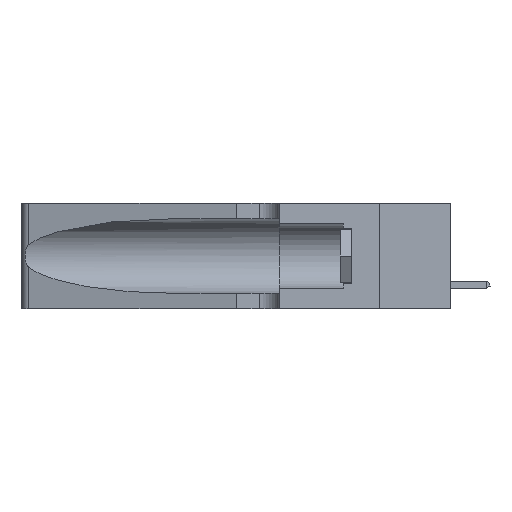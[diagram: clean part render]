
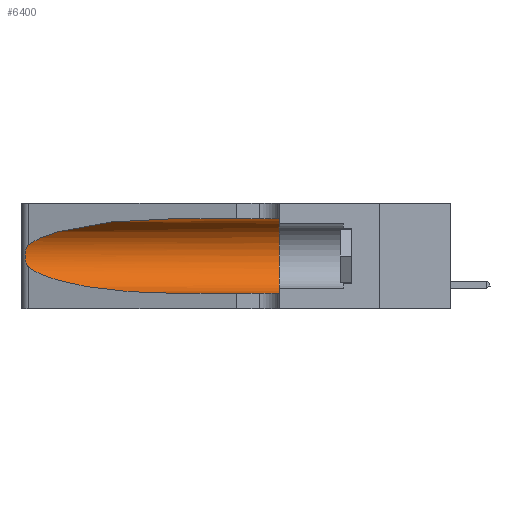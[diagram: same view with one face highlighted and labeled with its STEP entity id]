
A CAD part, left-side view. The second image highlights one B-rep face of the part: STEP entity #6400.
In plain terms, the highlighted cylindrical face has radius 3.308 mm (diameter 6.617 mm), a partial arc.
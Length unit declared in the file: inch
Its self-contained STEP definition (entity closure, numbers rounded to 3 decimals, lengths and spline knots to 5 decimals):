
#221 = CARTESIAN_POINT ( 'NONE',  ( 0.25555, 1.22993, 0.14849 ) ) ;
#281 = CARTESIAN_POINT ( 'NONE',  ( 0.25487, 1.22718, 0.22369 ) ) ;
#1464 = CARTESIAN_POINT ( 'NONE',  ( 0.25789, 1.23486, 0.15765 ) ) ;
#1633 = ORIENTED_EDGE ( 'NONE', *, *, #9034, .F. ) ;
#2254 = ORIENTED_EDGE ( 'NONE', *, *, #24382, .T. ) ;
#2431 = FACE_OUTER_BOUND ( 'NONE', #9905, .T. ) ;
#2759 = CARTESIAN_POINT ( 'NONE',  ( 0.1305, 1.61858, 0.185 ) ) ;
#3121 = CARTESIAN_POINT ( 'NONE',  ( 0.25555, 1.22994, 0.2215 ) ) ;
#3307 = CARTESIAN_POINT ( 'NONE',  ( 0.25487, 1.22718, 0.14631 ) ) ;
#3763 = CARTESIAN_POINT ( 'NONE',  ( 0.1305, 0.35, 0.185 ) ) ;
#4084 = DIRECTION ( 'NONE',  ( 0., 0., 1. ) ) ;
#4556 = CIRCLE ( 'NONE', #17474, 0.13025 ) ;
#5020 = CARTESIAN_POINT ( 'NONE',  ( 0.1305, 0.72297, 0.05475 ) ) ;
#5249 = CARTESIAN_POINT ( 'NONE',  ( 0.1305, 0.35, 0.05475 ) ) ;
#5495 = CARTESIAN_POINT ( 'NONE',  ( 0.25487, 1.22718, 0.14631 ) ) ;
#5517 = CARTESIAN_POINT ( 'NONE',  ( 0.26018, 1.23835, 0.19895 ) ) ;
#5883 = VECTOR ( 'NONE', #8369, 39.37008 ) ;
#6400 = ADVANCED_FACE ( 'NONE', ( #2431 ), #17748, .F. ) ;
#6982 = VERTEX_POINT ( 'NONE', #11121 ) ;
#7361 = CARTESIAN_POINT ( 'NONE',  ( 0.26075, 1.23896, 0.178 ) ) ;
#7892 = DIRECTION ( 'NONE',  ( 0., 0., -1. ) ) ;
#8369 = DIRECTION ( 'NONE',  ( 0., -1., 0. ) ) ;
#8412 = B_SPLINE_CURVE_WITH_KNOTS ( 'NONE', 3,
 ( #9029, #3121, #15159, #21361, #15250, #5517, #21276, #7361, #9299, #23348, #1464, #19436, #221, #14175 ),
 .UNSPECIFIED., .F., .F.,
 ( 4, 2, 2, 2, 2, 2, 4 ),
 ( 0., 0.00027, 0.00053, 0.00107, 0.0016, 0.00187, 0.00214 ),
 .UNSPECIFIED. ) ;
#8952 = AXIS2_PLACEMENT_3D ( 'NONE', #2759, #19678, #7892 ) ;
#9029 = CARTESIAN_POINT ( 'NONE',  ( 0.25487, 1.22718, 0.22369 ) ) ;
#9034 = EDGE_CURVE ( 'NONE', #14040, #11850, #11253, .T. ) ;
#9122 = DIRECTION ( 'NONE',  ( 0., -1., 0. ) ) ;
#9146 = ORIENTED_EDGE ( 'NONE', *, *, #11570, .T. ) ;
#9299 = CARTESIAN_POINT ( 'NONE',  ( 0.26017, 1.23833, 0.17102 ) ) ;
#9905 = EDGE_LOOP ( 'NONE', ( #9146, #12554, #13855, #2254, #18506, #1633 ) ) ;
#10214 = CARTESIAN_POINT ( 'NONE',  ( 0.25487, 1.22718, 0.22369 ) ) ;
#10729 =( BOUNDED_CURVE ( )  B_SPLINE_CURVE ( 3, ( #3307, #12988, #15086, #5020 ),
 .UNSPECIFIED., .F., .F. ) 
 B_SPLINE_CURVE_WITH_KNOTS ( ( 4, 4 ),
 ( 3.44316, 4.71239 ),
 .UNSPECIFIED. ) 
 CURVE ( )  GEOMETRIC_REPRESENTATION_ITEM ( )  RATIONAL_B_SPLINE_CURVE ( ( 1., 0.87, 0.87, 1. ) ) 
 REPRESENTATION_ITEM ( '' )  );
#11121 = CARTESIAN_POINT ( 'NONE',  ( 0.1305, 0.72297, 0.05475 ) ) ;
#11253 = LINE ( 'NONE', #12695, #5883 ) ;
#11570 = EDGE_CURVE ( 'NONE', #14040, #15154, #24263, .T. ) ;
#11850 = VERTEX_POINT ( 'NONE', #13913 ) ;
#12020 = DIRECTION ( 'NONE',  ( 0., 1., 0. ) ) ;
#12554 = ORIENTED_EDGE ( 'NONE', *, *, #19641, .T. ) ;
#12559 = VECTOR ( 'NONE', #9122, 39.37008 ) ;
#12693 = CARTESIAN_POINT ( 'NONE',  ( 0.18966, 0.96281, 0.31525 ) ) ;
#12695 = CARTESIAN_POINT ( 'NONE',  ( 0.1305, 1.61858, 0.31525 ) ) ;
#12988 = CARTESIAN_POINT ( 'NONE',  ( 0.2373, 1.15595, 0.08982 ) ) ;
#13855 = ORIENTED_EDGE ( 'NONE', *, *, #23455, .T. ) ;
#13913 = CARTESIAN_POINT ( 'NONE',  ( 0.1305, 0.35, 0.31525 ) ) ;
#14040 = VERTEX_POINT ( 'NONE', #14168 ) ;
#14168 = CARTESIAN_POINT ( 'NONE',  ( 0.1305, 0.72297, 0.31525 ) ) ;
#14175 = CARTESIAN_POINT ( 'NONE',  ( 0.25487, 1.22718, 0.14631 ) ) ;
#15086 = CARTESIAN_POINT ( 'NONE',  ( 0.18966, 0.96281, 0.05475 ) ) ;
#15087 = LINE ( 'NONE', #21468, #12559 ) ;
#15154 = VERTEX_POINT ( 'NONE', #10214 ) ;
#15159 = CARTESIAN_POINT ( 'NONE',  ( 0.25639, 1.23184, 0.21858 ) ) ;
#15250 = CARTESIAN_POINT ( 'NONE',  ( 0.25854, 1.2359, 0.20912 ) ) ;
#15764 = CARTESIAN_POINT ( 'NONE',  ( 0.2373, 1.15595, 0.28018 ) ) ;
#16362 = CARTESIAN_POINT ( 'NONE',  ( 0.1305, 0.72297, 0.31525 ) ) ;
#16841 = VERTEX_POINT ( 'NONE', #5495 ) ;
#17474 = AXIS2_PLACEMENT_3D ( 'NONE', #3763, #12020, #4084 ) ;
#17748 = CYLINDRICAL_SURFACE ( 'NONE', #8952, 0.13025 ) ;
#18506 = ORIENTED_EDGE ( 'NONE', *, *, #22200, .F. ) ;
#19436 = CARTESIAN_POINT ( 'NONE',  ( 0.25639, 1.23186, 0.15144 ) ) ;
#19641 = EDGE_CURVE ( 'NONE', #15154, #16841, #8412, .T. ) ;
#19678 = DIRECTION ( 'NONE',  ( 0., -1., 0. ) ) ;
#21276 = CARTESIAN_POINT ( 'NONE',  ( 0.26075, 1.23896, 0.19203 ) ) ;
#21361 = CARTESIAN_POINT ( 'NONE',  ( 0.25787, 1.23484, 0.2124 ) ) ;
#21468 = CARTESIAN_POINT ( 'NONE',  ( 0.1305, 1.61858, 0.05475 ) ) ;
#22200 = EDGE_CURVE ( 'NONE', #11850, #25116, #4556, .T. ) ;
#23348 = CARTESIAN_POINT ( 'NONE',  ( 0.25856, 1.23593, 0.16098 ) ) ;
#23455 = EDGE_CURVE ( 'NONE', #16841, #6982, #10729, .T. ) ;
#24263 =( BOUNDED_CURVE ( )  B_SPLINE_CURVE ( 3, ( #16362, #12693, #15764, #281 ),
 .UNSPECIFIED., .F., .T. ) 
 B_SPLINE_CURVE_WITH_KNOTS ( ( 4, 4 ),
 ( 1.5708, 2.84003 ),
 .UNSPECIFIED. ) 
 CURVE ( )  GEOMETRIC_REPRESENTATION_ITEM ( )  RATIONAL_B_SPLINE_CURVE ( ( 1., 0.87, 0.87, 1. ) ) 
 REPRESENTATION_ITEM ( '' )  );
#24382 = EDGE_CURVE ( 'NONE', #6982, #25116, #15087, .T. ) ;
#25116 = VERTEX_POINT ( 'NONE', #5249 ) ;
